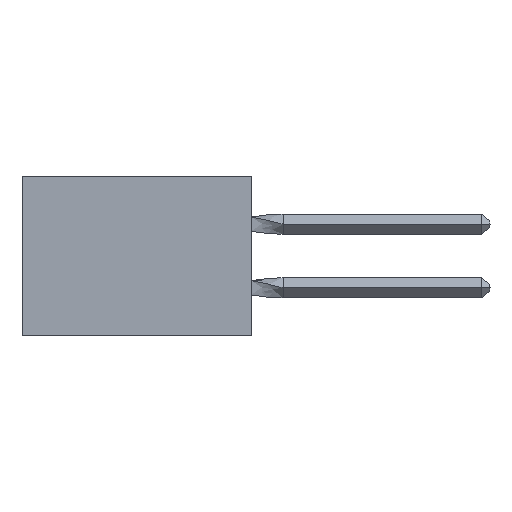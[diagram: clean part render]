
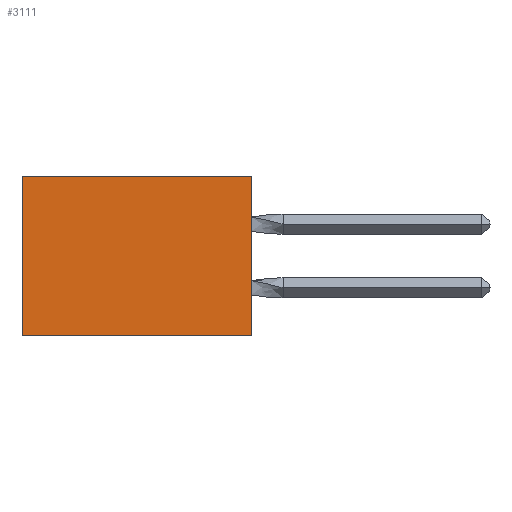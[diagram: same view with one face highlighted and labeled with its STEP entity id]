
A CAD part, left-side view. The second image highlights one B-rep face of the part: STEP entity #3111.
In plain terms, the highlighted planar face has unit normal (-1, 0, 0).
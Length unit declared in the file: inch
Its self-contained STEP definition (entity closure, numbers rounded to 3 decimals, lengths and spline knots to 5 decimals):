
#1117 = EDGE_CURVE ( 'NONE', #23206, #24615, #18320, .T. ) ;
#1289 = EDGE_CURVE ( 'NONE', #17648, #23206, #1967, .T. ) ;
#1651 = VECTOR ( 'NONE', #13711, 39.37008 ) ;
#1967 = LINE ( 'NONE', #27615, #2667 ) ;
#2667 = VECTOR ( 'NONE', #10760, 39.37008 ) ;
#3111 = ADVANCED_FACE ( 'NONE', ( #6542 ), #19010, .F. ) ;
#4290 = CARTESIAN_POINT ( 'NONE',  ( 0.305, 0., -0.5 ) ) ;
#5603 = DIRECTION ( 'NONE',  ( 0., 0., -1. ) ) ;
#6251 = DIRECTION ( 'NONE',  ( 1., 0., 0. ) ) ;
#6542 = FACE_OUTER_BOUND ( 'NONE', #22412, .T. ) ;
#7958 = DIRECTION ( 'NONE',  ( 0., 0., -1. ) ) ;
#8163 = ORIENTED_EDGE ( 'NONE', *, *, #10397, .F. ) ;
#9181 = CARTESIAN_POINT ( 'NONE',  ( 0.305, 0.72, 0. ) ) ;
#9795 = VECTOR ( 'NONE', #5603, 39.37008 ) ;
#10397 = EDGE_CURVE ( 'NONE', #17648, #21934, #10451, .T. ) ;
#10451 = LINE ( 'NONE', #22747, #9795 ) ;
#10760 = DIRECTION ( 'NONE',  ( 0., 1., 0. ) ) ;
#12825 = ORIENTED_EDGE ( 'NONE', *, *, #1289, .T. ) ;
#12988 = LINE ( 'NONE', #15687, #1651 ) ;
#13711 = DIRECTION ( 'NONE',  ( 0., 1., 0. ) ) ;
#15687 = CARTESIAN_POINT ( 'NONE',  ( 0.305, 0., -0.5 ) ) ;
#17648 = VERTEX_POINT ( 'NONE', #17913 ) ;
#17913 = CARTESIAN_POINT ( 'NONE',  ( 0.305, 0., 0. ) ) ;
#18320 = LINE ( 'NONE', #20693, #25325 ) ;
#18833 = ORIENTED_EDGE ( 'NONE', *, *, #1117, .T. ) ;
#19010 = PLANE ( 'NONE',  #19255 ) ;
#19255 = AXIS2_PLACEMENT_3D ( 'NONE', #4290, #6251, #25455 ) ;
#20693 = CARTESIAN_POINT ( 'NONE',  ( 0.305, 0.72, -0.5 ) ) ;
#21934 = VERTEX_POINT ( 'NONE', #23186 ) ;
#22412 = EDGE_LOOP ( 'NONE', ( #18833, #27130, #8163, #12825 ) ) ;
#22747 = CARTESIAN_POINT ( 'NONE',  ( 0.305, 0., -0.5 ) ) ;
#23186 = CARTESIAN_POINT ( 'NONE',  ( 0.305, 0., -0.5 ) ) ;
#23206 = VERTEX_POINT ( 'NONE', #9181 ) ;
#23666 = CARTESIAN_POINT ( 'NONE',  ( 0.305, 0.72, -0.5 ) ) ;
#24615 = VERTEX_POINT ( 'NONE', #23666 ) ;
#25325 = VECTOR ( 'NONE', #7958, 39.37008 ) ;
#25455 = DIRECTION ( 'NONE',  ( 0., 0., -1. ) ) ;
#26965 = EDGE_CURVE ( 'NONE', #21934, #24615, #12988, .T. ) ;
#27130 = ORIENTED_EDGE ( 'NONE', *, *, #26965, .F. ) ;
#27615 = CARTESIAN_POINT ( 'NONE',  ( 0.305, 0., 0. ) ) ;
